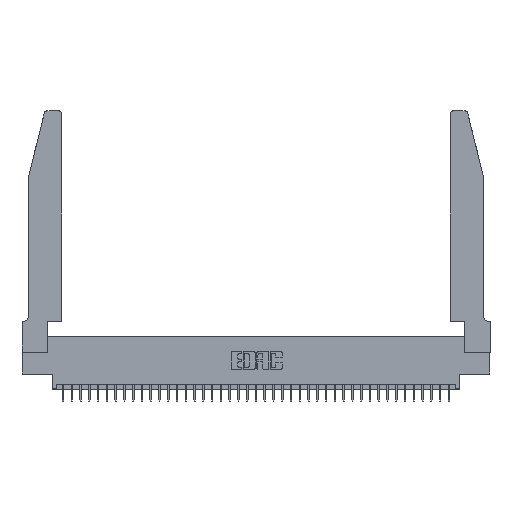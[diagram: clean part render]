
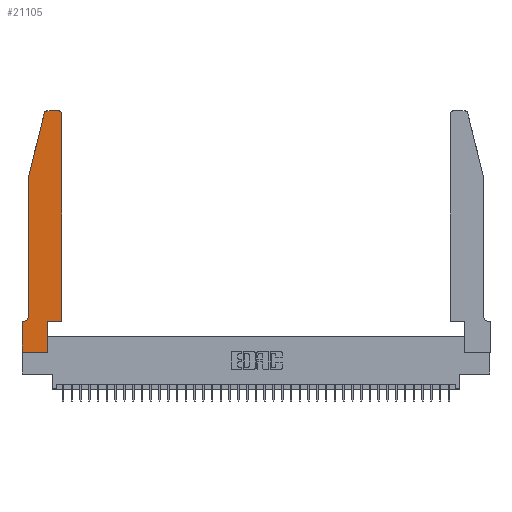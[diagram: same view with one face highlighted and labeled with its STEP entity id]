
A CAD part, top view. The second image highlights one B-rep face of the part: STEP entity #21105.
In plain terms, the highlighted planar face has unit normal (0, 0, 1).
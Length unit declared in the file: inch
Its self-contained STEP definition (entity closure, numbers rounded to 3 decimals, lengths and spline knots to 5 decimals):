
#230 = CARTESIAN_POINT ( 'NONE',  ( 0.2605, 2.75, 0.37 ) ) ;
#403 = VECTOR ( 'NONE', #18192, 39.37008 ) ;
#755 = CARTESIAN_POINT ( 'NONE',  ( 0.0755, 0.35, 0.37 ) ) ;
#877 = LINE ( 'NONE', #22288, #24728 ) ;
#1347 = VERTEX_POINT ( 'NONE', #34003 ) ;
#1402 = ORIENTED_EDGE ( 'NONE', *, *, #37441, .T. ) ;
#1814 = AXIS2_PLACEMENT_3D ( 'NONE', #31776, #21894, #4122 ) ;
#1946 = FACE_OUTER_BOUND ( 'NONE', #30202, .T. ) ;
#1976 = CARTESIAN_POINT ( 'NONE',  ( 0., 0.35, 0.37 ) ) ;
#2533 = DIRECTION ( 'NONE',  ( 1., 0., 0. ) ) ;
#3036 = DIRECTION ( 'NONE',  ( 0., -1., 0. ) ) ;
#3767 = LINE ( 'NONE', #12849, #19955 ) ;
#4122 = DIRECTION ( 'NONE',  ( -1., 0., 0. ) ) ;
#4192 = EDGE_CURVE ( 'NONE', #17576, #14986, #3767, .T. ) ;
#4524 = LINE ( 'NONE', #29141, #13686 ) ;
#4766 = VECTOR ( 'NONE', #3036, 39.37008 ) ;
#4831 = EDGE_CURVE ( 'NONE', #1347, #35370, #8947, .T. ) ;
#6413 = DIRECTION ( 'NONE',  ( -0.239, -0.971, 0. ) ) ;
#6808 = CARTESIAN_POINT ( 'NONE',  ( 0.0755, 2., 0.37 ) ) ;
#7771 = ORIENTED_EDGE ( 'NONE', *, *, #11478, .T. ) ;
#8013 = EDGE_CURVE ( 'NONE', #36557, #31168, #23170, .T. ) ;
#8121 = AXIS2_PLACEMENT_3D ( 'NONE', #32427, #17868, #2533 ) ;
#8325 = DIRECTION ( 'NONE',  ( 1., 0., 0. ) ) ;
#8947 = LINE ( 'NONE', #39834, #11626 ) ;
#9512 = VERTEX_POINT ( 'NONE', #12435 ) ;
#9556 = ORIENTED_EDGE ( 'NONE', *, *, #14782, .T. ) ;
#9708 = VERTEX_POINT ( 'NONE', #35029 ) ;
#11478 = EDGE_CURVE ( 'NONE', #9708, #35748, #38820, .T. ) ;
#11581 = CARTESIAN_POINT ( 'NONE',  ( 0.4205, 2.72, 0.37 ) ) ;
#11626 = VECTOR ( 'NONE', #11976, 39.37008 ) ;
#11631 = PLANE ( 'NONE',  #8121 ) ;
#11976 = DIRECTION ( 'NONE',  ( 0., 1., 0. ) ) ;
#12435 = CARTESIAN_POINT ( 'NONE',  ( 0.284, 2.75, 0.37 ) ) ;
#12639 = VECTOR ( 'NONE', #8325, 39.37008 ) ;
#12849 = CARTESIAN_POINT ( 'NONE',  ( 0.0755, 2., 0.37 ) ) ;
#13073 = EDGE_CURVE ( 'NONE', #35654, #9512, #27885, .T. ) ;
#13245 = CARTESIAN_POINT ( 'NONE',  ( 0.0755, 2., 0.37 ) ) ;
#13686 = VECTOR ( 'NONE', #13801, 39.37008 ) ;
#13801 = DIRECTION ( 'NONE',  ( 0., 1., 0. ) ) ;
#14530 = EDGE_CURVE ( 'NONE', #14986, #36557, #35339, .T. ) ;
#14782 = EDGE_CURVE ( 'NONE', #35370, #35654, #20205, .T. ) ;
#14820 = ORIENTED_EDGE ( 'NONE', *, *, #17330, .T. ) ;
#14986 = VERTEX_POINT ( 'NONE', #31132 ) ;
#16878 = DIRECTION ( 'NONE',  ( -1., 0., 0. ) ) ;
#17330 = EDGE_CURVE ( 'NONE', #23336, #1347, #877, .T. ) ;
#17576 = VERTEX_POINT ( 'NONE', #13245 ) ;
#17623 = AXIS2_PLACEMENT_3D ( 'NONE', #11581, #23890, #39847 ) ;
#17868 = DIRECTION ( 'NONE',  ( 0., 0., 1. ) ) ;
#18192 = DIRECTION ( 'NONE',  ( -1., 0., 0. ) ) ;
#19218 = ORIENTED_EDGE ( 'NONE', *, *, #4831, .T. ) ;
#19646 = DIRECTION ( 'NONE',  ( 1., 0., 0. ) ) ;
#19955 = VECTOR ( 'NONE', #25165, 39.37008 ) ;
#20205 = CIRCLE ( 'NONE', #17623, 0.03 ) ;
#20577 = CARTESIAN_POINT ( 'NONE',  ( 0.2865, 0.35, 0.37 ) ) ;
#20649 = EDGE_CURVE ( 'NONE', #28066, #17576, #36913, .T. ) ;
#21105 = ADVANCED_FACE ( 'NONE', ( #1946 ), #11631, .T. ) ;
#21637 = CARTESIAN_POINT ( 'NONE',  ( 0.2865, 0., 0.37 ) ) ;
#21665 = VECTOR ( 'NONE', #6413, 39.37008 ) ;
#21894 = DIRECTION ( 'NONE',  ( 0., 0., -1. ) ) ;
#22288 = CARTESIAN_POINT ( 'NONE',  ( 0.4505, 0.35, 0.37 ) ) ;
#22988 = ORIENTED_EDGE ( 'NONE', *, *, #38000, .T. ) ;
#23170 = LINE ( 'NONE', #755, #26622 ) ;
#23336 = VERTEX_POINT ( 'NONE', #20577 ) ;
#23833 = CARTESIAN_POINT ( 'NONE',  ( 0., 0., 0.37 ) ) ;
#23890 = DIRECTION ( 'NONE',  ( 0., 0., 1. ) ) ;
#24135 = AXIS2_PLACEMENT_3D ( 'NONE', #38646, #25917, #19646 ) ;
#24728 = VECTOR ( 'NONE', #38038, 39.37008 ) ;
#25165 = DIRECTION ( 'NONE',  ( 0., -1., 0. ) ) ;
#25917 = DIRECTION ( 'NONE',  ( 0., 0., 1. ) ) ;
#26622 = VECTOR ( 'NONE', #16878, 39.37008 ) ;
#27089 = CARTESIAN_POINT ( 'NONE',  ( 0.4205, 2.75, 0.37 ) ) ;
#27885 = LINE ( 'NONE', #230, #403 ) ;
#28066 = VERTEX_POINT ( 'NONE', #30659 ) ;
#28320 = ORIENTED_EDGE ( 'NONE', *, *, #14530, .T. ) ;
#28646 = CIRCLE ( 'NONE', #24135, 0.03 ) ;
#29141 = CARTESIAN_POINT ( 'NONE',  ( 0.2865, 0.35, 0.37 ) ) ;
#30202 = EDGE_LOOP ( 'NONE', ( #34971, #22988, #35671, #38325, #28320, #35146, #1402, #7771, #37138, #14820, #19218, #9556 ) ) ;
#30659 = CARTESIAN_POINT ( 'NONE',  ( 0.25487, 2.72718, 0.37 ) ) ;
#30689 = LINE ( 'NONE', #23833, #4766 ) ;
#31132 = CARTESIAN_POINT ( 'NONE',  ( 0.0755, 0.42, 0.37 ) ) ;
#31168 = VERTEX_POINT ( 'NONE', #1976 ) ;
#31776 = CARTESIAN_POINT ( 'NONE',  ( 0.0055, 0.42, 0.37 ) ) ;
#32427 = CARTESIAN_POINT ( 'NONE',  ( 0., 0.35, 0.37 ) ) ;
#33360 = EDGE_CURVE ( 'NONE', #35748, #23336, #4524, .T. ) ;
#34003 = CARTESIAN_POINT ( 'NONE',  ( 0.4505, 0.35, 0.37 ) ) ;
#34971 = ORIENTED_EDGE ( 'NONE', *, *, #13073, .T. ) ;
#35029 = CARTESIAN_POINT ( 'NONE',  ( 0., 0., 0.37 ) ) ;
#35146 = ORIENTED_EDGE ( 'NONE', *, *, #8013, .T. ) ;
#35339 = CIRCLE ( 'NONE', #1814, 0.07 ) ;
#35370 = VERTEX_POINT ( 'NONE', #37830 ) ;
#35654 = VERTEX_POINT ( 'NONE', #27089 ) ;
#35671 = ORIENTED_EDGE ( 'NONE', *, *, #20649, .T. ) ;
#35748 = VERTEX_POINT ( 'NONE', #21637 ) ;
#36557 = VERTEX_POINT ( 'NONE', #37483 ) ;
#36913 = LINE ( 'NONE', #6808, #21665 ) ;
#37138 = ORIENTED_EDGE ( 'NONE', *, *, #33360, .T. ) ;
#37441 = EDGE_CURVE ( 'NONE', #31168, #9708, #30689, .T. ) ;
#37483 = CARTESIAN_POINT ( 'NONE',  ( 0.0055, 0.35, 0.37 ) ) ;
#37830 = CARTESIAN_POINT ( 'NONE',  ( 0.4505, 2.72, 0.37 ) ) ;
#38000 = EDGE_CURVE ( 'NONE', #9512, #28066, #28646, .T. ) ;
#38038 = DIRECTION ( 'NONE',  ( 1., 0., 0. ) ) ;
#38325 = ORIENTED_EDGE ( 'NONE', *, *, #4192, .T. ) ;
#38416 = CARTESIAN_POINT ( 'NONE',  ( 0., 0., 0.37 ) ) ;
#38646 = CARTESIAN_POINT ( 'NONE',  ( 0.284, 2.72, 0.37 ) ) ;
#38820 = LINE ( 'NONE', #38416, #12639 ) ;
#39834 = CARTESIAN_POINT ( 'NONE',  ( 0.4505, 0.35, 0.37 ) ) ;
#39847 = DIRECTION ( 'NONE',  ( 1., 0., 0. ) ) ;
